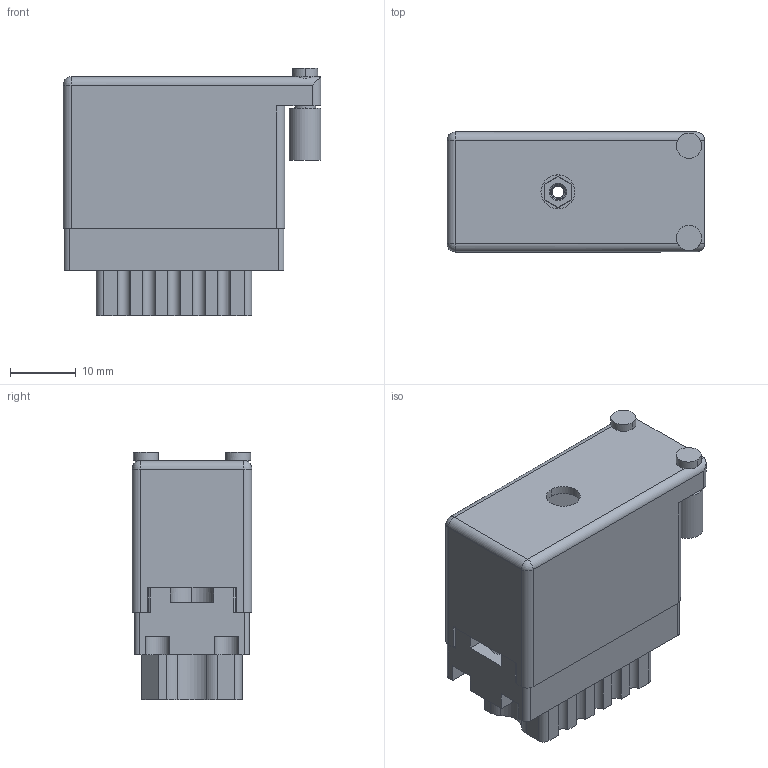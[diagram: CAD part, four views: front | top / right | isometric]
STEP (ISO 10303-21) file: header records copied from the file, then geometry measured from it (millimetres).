
FILE_DESCRIPTION (( 'STEP AP203' ), '1' );
FILE_NAME ('519-014-520-456.STEP', '2020-09-09T19:17:24', ( '' ), ( '' ), 'SwSTEP 2.0', 'SolidWorks 2020', '' );
FILE_SCHEMA (( 'CONFIG_CONTROL_DESIGN' ));
Length unit declared in the file: inch
Products named in the file (5): 516-230-001_Metal - 020 Side Entry; 516-252-025-100_516-252-025-100; 519 Receptacle Insulator_014; 519-014-520-456; 516-292-001_520 Contact
Assembly tree (17 placements, depth 2):
  519-014-520-456
    519 Receptacle Insulator_014
    516-292-001_520 Contact  x14
    516-252-025-100_516-252-025-100
    516-230-001_Metal - 020 Side Entry
Bounding box: 39.12 x 18.16 x 37.52 mm (x, y, z)
Volume: 10434.9 mm3; surface area: 15253.3 mm2
Topology: 17 solids, 17 shells, 1607 faces, 4634 edges, 3069 vertices
Faces by surface type: plane 955, cylinder 552, bspline 87, cone 11, sphere 2
Entity records: 25766 total; most frequent: CARTESIAN_POINT 6932, ORIENTED_EDGE 3856, DIRECTION 3693, EDGE_CURVE 1928, VECTOR 1337, LINE 1337, VERTEX_POINT 1275, AXIS2_PLACEMENT_3D 1178
